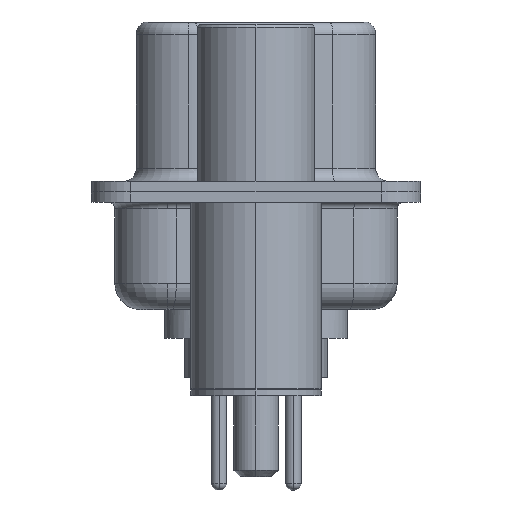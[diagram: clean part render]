
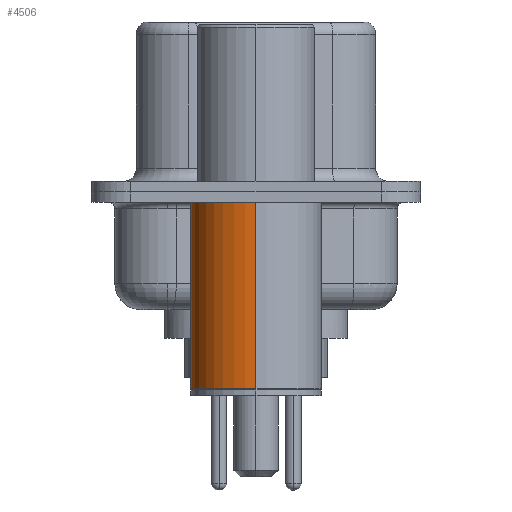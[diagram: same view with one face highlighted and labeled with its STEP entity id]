
A CAD part, left-side view. The second image highlights one B-rep face of the part: STEP entity #4506.
In plain terms, the highlighted cylindrical face has radius 2.5 mm (diameter 5 mm), a partial arc.
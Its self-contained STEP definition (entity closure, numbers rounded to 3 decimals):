
#249 = CIRCLE ( 'NONE', #6360, 2.5 ) ;
#772 = CARTESIAN_POINT ( 'NONE',  ( 0., 0., -7.525 ) ) ;
#844 = DIRECTION ( 'NONE',  ( 0., 0., 1. ) ) ;
#1508 = LINE ( 'NONE', #11415, #8779 ) ;
#2483 = FACE_OUTER_BOUND ( 'NONE', #10086, .T. ) ;
#2718 = CARTESIAN_POINT ( 'NONE',  ( 0., 0., 0.581 ) ) ;
#3038 = ORIENTED_EDGE ( 'NONE', *, *, #15004, .F. ) ;
#4320 = CARTESIAN_POINT ( 'NONE',  ( 2.5, 0., -7.525 ) ) ;
#4506 = ADVANCED_FACE ( 'NONE', ( #2483 ), #15910, .T. ) ;
#5076 = CARTESIAN_POINT ( 'NONE',  ( -2.5, 0., 0.581 ) ) ;
#5140 = ORIENTED_EDGE ( 'NONE', *, *, #6680, .T. ) ;
#6049 = DIRECTION ( 'NONE',  ( 1., 0., 0. ) ) ;
#6236 = CARTESIAN_POINT ( 'NONE',  ( 2.5, 0., -0.4 ) ) ;
#6360 = AXIS2_PLACEMENT_3D ( 'NONE', #17906, #17743, #16041 ) ;
#6422 = DIRECTION ( 'NONE',  ( 0., 0., 1. ) ) ;
#6680 = EDGE_CURVE ( 'NONE', #7696, #15797, #8619, .T. ) ;
#7415 = DIRECTION ( 'NONE',  ( 1., 0., 0. ) ) ;
#7696 = VERTEX_POINT ( 'NONE', #4320 ) ;
#8116 = DIRECTION ( 'NONE',  ( 0., 0., 1. ) ) ;
#8140 = EDGE_CURVE ( 'NONE', #15797, #15323, #19590, .T. ) ;
#8619 = CIRCLE ( 'NONE', #19844, 2.5 ) ;
#8779 = VECTOR ( 'NONE', #6422, 1000. ) ;
#9076 = VECTOR ( 'NONE', #8116, 1000. ) ;
#10086 = EDGE_LOOP ( 'NONE', ( #5140, #17098, #14299, #3038 ) ) ;
#11415 = CARTESIAN_POINT ( 'NONE',  ( 2.5, 0., 0.581 ) ) ;
#11692 = CARTESIAN_POINT ( 'NONE',  ( -2.5, 0., -7.525 ) ) ;
#14282 = AXIS2_PLACEMENT_3D ( 'NONE', #2718, #15914, #6049 ) ;
#14299 = ORIENTED_EDGE ( 'NONE', *, *, #19412, .F. ) ;
#15004 = EDGE_CURVE ( 'NONE', #7696, #17221, #1508, .T. ) ;
#15323 = VERTEX_POINT ( 'NONE', #21228 ) ;
#15797 = VERTEX_POINT ( 'NONE', #11692 ) ;
#15910 = CYLINDRICAL_SURFACE ( 'NONE', #14282, 2.5 ) ;
#15914 = DIRECTION ( 'NONE',  ( 0., 0., 1. ) ) ;
#16041 = DIRECTION ( 'NONE',  ( 1., 0., 0. ) ) ;
#17098 = ORIENTED_EDGE ( 'NONE', *, *, #8140, .T. ) ;
#17221 = VERTEX_POINT ( 'NONE', #6236 ) ;
#17743 = DIRECTION ( 'NONE',  ( 0., 0., 1. ) ) ;
#17906 = CARTESIAN_POINT ( 'NONE',  ( 0., 0., -0.4 ) ) ;
#19412 = EDGE_CURVE ( 'NONE', #17221, #15323, #249, .T. ) ;
#19590 = LINE ( 'NONE', #5076, #9076 ) ;
#19844 = AXIS2_PLACEMENT_3D ( 'NONE', #772, #844, #7415 ) ;
#21228 = CARTESIAN_POINT ( 'NONE',  ( -2.5, 0., -0.4 ) ) ;
